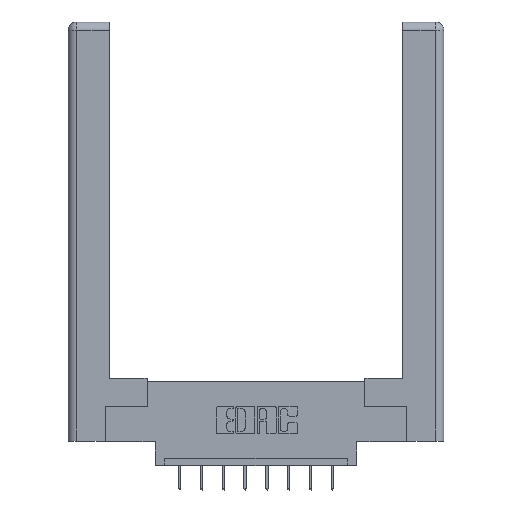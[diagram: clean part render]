
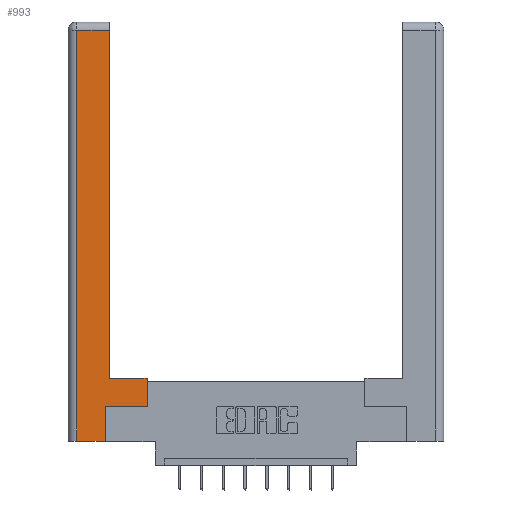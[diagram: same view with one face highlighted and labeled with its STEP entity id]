
A CAD part, top view. The second image highlights one B-rep face of the part: STEP entity #993.
In plain terms, the highlighted planar face has unit normal (0, 0, 1).
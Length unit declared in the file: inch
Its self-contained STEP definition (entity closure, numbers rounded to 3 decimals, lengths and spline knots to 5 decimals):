
#437 = LINE ( 'NONE', #8481, #6189 ) ;
#600 = VERTEX_POINT ( 'NONE', #4426 ) ;
#848 = CARTESIAN_POINT ( 'NONE',  ( 0.295, 0.45, 0. ) ) ;
#993 = ADVANCED_FACE ( 'NONE', ( #1130 ), #9606, .F. ) ;
#1130 = FACE_OUTER_BOUND ( 'NONE', #8133, .T. ) ;
#1155 = DIRECTION ( 'NONE',  ( 0., 1., 0. ) ) ;
#1385 = DIRECTION ( 'NONE',  ( 0., 1., 0. ) ) ;
#1440 = LINE ( 'NONE', #11740, #11003 ) ;
#1452 = EDGE_CURVE ( 'NONE', #600, #5827, #9261, .T. ) ;
#2068 = CARTESIAN_POINT ( 'NONE',  ( 0.0615, 0., 0. ) ) ;
#2218 = ORIENTED_EDGE ( 'NONE', *, *, #9054, .T. ) ;
#2506 = CARTESIAN_POINT ( 'NONE',  ( 0.0615, 0., 0. ) ) ;
#2571 = VERTEX_POINT ( 'NONE', #12617 ) ;
#2868 = ORIENTED_EDGE ( 'NONE', *, *, #10495, .T. ) ;
#3488 = DIRECTION ( 'NONE',  ( 0., 0., -1. ) ) ;
#3817 = VECTOR ( 'NONE', #9114, 39.37008 ) ;
#4070 = ORIENTED_EDGE ( 'NONE', *, *, #11140, .T. ) ;
#4332 = CARTESIAN_POINT ( 'NONE',  ( 0.565, 0.245, 0. ) ) ;
#4426 = CARTESIAN_POINT ( 'NONE',  ( 0.565, 0.245, 0. ) ) ;
#4537 = VECTOR ( 'NONE', #1155, 39.37008 ) ;
#4559 = VERTEX_POINT ( 'NONE', #2506 ) ;
#4644 = CARTESIAN_POINT ( 'NONE',  ( 0.0615, 2.94, 0. ) ) ;
#4914 = AXIS2_PLACEMENT_3D ( 'NONE', #9560, #3488, #6611 ) ;
#5400 = VERTEX_POINT ( 'NONE', #7299 ) ;
#5827 = VERTEX_POINT ( 'NONE', #8905 ) ;
#5828 = ORIENTED_EDGE ( 'NONE', *, *, #8404, .T. ) ;
#6189 = VECTOR ( 'NONE', #6440, 39.37008 ) ;
#6438 = VERTEX_POINT ( 'NONE', #9094 ) ;
#6440 = DIRECTION ( 'NONE',  ( -1., 0., 0. ) ) ;
#6611 = DIRECTION ( 'NONE',  ( -1., 0., 0. ) ) ;
#6618 = VECTOR ( 'NONE', #12276, 39.37008 ) ;
#6742 = EDGE_CURVE ( 'NONE', #4559, #6438, #1440, .T. ) ;
#6777 = CARTESIAN_POINT ( 'NONE',  ( 0.565, 0.45, 0. ) ) ;
#6932 = VECTOR ( 'NONE', #9437, 39.37008 ) ;
#7167 = ORIENTED_EDGE ( 'NONE', *, *, #1452, .T. ) ;
#7242 = LINE ( 'NONE', #12105, #4537 ) ;
#7299 = CARTESIAN_POINT ( 'NONE',  ( 0.295, 2.94, 0. ) ) ;
#7749 = LINE ( 'NONE', #2068, #6618 ) ;
#8133 = EDGE_LOOP ( 'NONE', ( #4070, #5828, #12687, #9098, #13157, #2868, #7167, #2218 ) ) ;
#8156 = LINE ( 'NONE', #12738, #12887 ) ;
#8375 = EDGE_CURVE ( 'NONE', #6438, #10692, #8156, .T. ) ;
#8404 = EDGE_CURVE ( 'NONE', #5400, #2571, #13204, .T. ) ;
#8481 = CARTESIAN_POINT ( 'NONE',  ( 0.295, 0.45, 0. ) ) ;
#8905 = CARTESIAN_POINT ( 'NONE',  ( 0.565, 0.45, 0. ) ) ;
#9054 = EDGE_CURVE ( 'NONE', #5827, #10062, #437, .T. ) ;
#9094 = CARTESIAN_POINT ( 'NONE',  ( 0.265, 0., 0. ) ) ;
#9098 = ORIENTED_EDGE ( 'NONE', *, *, #6742, .T. ) ;
#9114 = DIRECTION ( 'NONE',  ( 0., 1., 0. ) ) ;
#9261 = LINE ( 'NONE', #6777, #3817 ) ;
#9437 = DIRECTION ( 'NONE',  ( 1., 0., 0. ) ) ;
#9560 = CARTESIAN_POINT ( 'NONE',  ( 0., 0., 0. ) ) ;
#9606 = PLANE ( 'NONE',  #4914 ) ;
#9818 = LINE ( 'NONE', #4332, #6932 ) ;
#9848 = DIRECTION ( 'NONE',  ( -1., 0., 0. ) ) ;
#10062 = VERTEX_POINT ( 'NONE', #848 ) ;
#10495 = EDGE_CURVE ( 'NONE', #10692, #600, #9818, .T. ) ;
#10650 = DIRECTION ( 'NONE',  ( 1., 0., 0. ) ) ;
#10692 = VERTEX_POINT ( 'NONE', #11438 ) ;
#10804 = EDGE_CURVE ( 'NONE', #2571, #4559, #7749, .T. ) ;
#11003 = VECTOR ( 'NONE', #10650, 39.37008 ) ;
#11140 = EDGE_CURVE ( 'NONE', #10062, #5400, #7242, .T. ) ;
#11438 = CARTESIAN_POINT ( 'NONE',  ( 0.265, 0.245, 0. ) ) ;
#11740 = CARTESIAN_POINT ( 'NONE',  ( 0.265, 0., 0. ) ) ;
#12105 = CARTESIAN_POINT ( 'NONE',  ( 0.295, 3., 0. ) ) ;
#12276 = DIRECTION ( 'NONE',  ( 0., -1., 0. ) ) ;
#12617 = CARTESIAN_POINT ( 'NONE',  ( 0.0615, 2.94, 0. ) ) ;
#12687 = ORIENTED_EDGE ( 'NONE', *, *, #10804, .T. ) ;
#12738 = CARTESIAN_POINT ( 'NONE',  ( 0.265, 0.245, 0. ) ) ;
#12887 = VECTOR ( 'NONE', #1385, 39.37008 ) ;
#13044 = VECTOR ( 'NONE', #9848, 39.37008 ) ;
#13157 = ORIENTED_EDGE ( 'NONE', *, *, #8375, .T. ) ;
#13204 = LINE ( 'NONE', #4644, #13044 ) ;
